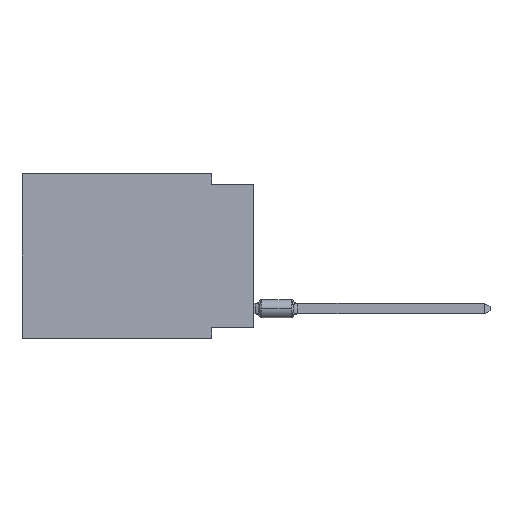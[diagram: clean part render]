
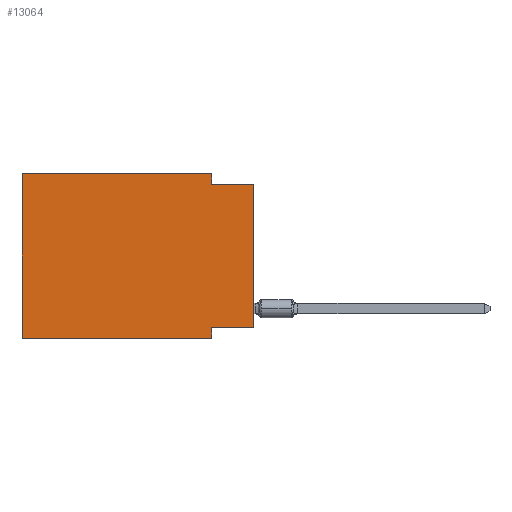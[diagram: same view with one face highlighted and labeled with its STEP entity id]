
A CAD part, left-side view. The second image highlights one B-rep face of the part: STEP entity #13064.
In plain terms, the highlighted planar face has unit normal (-1, 0, 0).
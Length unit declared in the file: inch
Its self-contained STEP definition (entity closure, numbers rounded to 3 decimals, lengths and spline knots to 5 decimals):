
#58 = VECTOR ( 'NONE', #435, 39.37008 ) ;
#290 = VECTOR ( 'NONE', #15337, 39.37008 ) ;
#435 = DIRECTION ( 'NONE',  ( 0., 0., -1. ) ) ;
#760 = DIRECTION ( 'NONE',  ( 0., 1., 0. ) ) ;
#1007 = DIRECTION ( 'NONE',  ( 0., -1., 0. ) ) ;
#1245 = ORIENTED_EDGE ( 'NONE', *, *, #11495, .T. ) ;
#1756 = ORIENTED_EDGE ( 'NONE', *, *, #4462, .F. ) ;
#1839 = DIRECTION ( 'NONE',  ( 0., 0., 1. ) ) ;
#2349 = LINE ( 'NONE', #4537, #13344 ) ;
#2824 = VECTOR ( 'NONE', #760, 39.37008 ) ;
#3099 = AXIS2_PLACEMENT_3D ( 'NONE', #5139, #9951, #13557 ) ;
#3325 = DIRECTION ( 'NONE',  ( 0., -1., 0. ) ) ;
#3511 = CARTESIAN_POINT ( 'NONE',  ( 0., 0.55, 0. ) ) ;
#4141 = ORIENTED_EDGE ( 'NONE', *, *, #4559, .F. ) ;
#4283 = CARTESIAN_POINT ( 'NONE',  ( 0., 0., -0.365 ) ) ;
#4462 = EDGE_CURVE ( 'NONE', #7658, #9899, #7679, .T. ) ;
#4537 = CARTESIAN_POINT ( 'NONE',  ( 0., 0.55, -0.39 ) ) ;
#4559 = EDGE_CURVE ( 'NONE', #5043, #13030, #5385, .T. ) ;
#4664 = ORIENTED_EDGE ( 'NONE', *, *, #12522, .F. ) ;
#5043 = VERTEX_POINT ( 'NONE', #10552 ) ;
#5113 = CARTESIAN_POINT ( 'NONE',  ( 0., 0., -0.025 ) ) ;
#5139 = CARTESIAN_POINT ( 'NONE',  ( 0., 0.55, 0. ) ) ;
#5385 = LINE ( 'NONE', #6409, #58 ) ;
#5472 = EDGE_LOOP ( 'NONE', ( #7021, #10696, #1756, #10956, #4664, #1245, #4141, #13862 ) ) ;
#5552 = VERTEX_POINT ( 'NONE', #8340 ) ;
#5589 = VECTOR ( 'NONE', #3325, 39.37008 ) ;
#6409 = CARTESIAN_POINT ( 'NONE',  ( 0., 0.1, -0.39 ) ) ;
#6539 = LINE ( 'NONE', #10310, #8101 ) ;
#6555 = CARTESIAN_POINT ( 'NONE',  ( 0., 0.55, 0. ) ) ;
#6660 = EDGE_CURVE ( 'NONE', #5552, #8252, #12189, .T. ) ;
#6736 = CARTESIAN_POINT ( 'NONE',  ( 0., 0.55, -0.39 ) ) ;
#7006 = VECTOR ( 'NONE', #14533, 39.37008 ) ;
#7021 = ORIENTED_EDGE ( 'NONE', *, *, #6660, .T. ) ;
#7084 = LINE ( 'NONE', #12830, #290 ) ;
#7658 = VERTEX_POINT ( 'NONE', #14203 ) ;
#7679 = LINE ( 'NONE', #7983, #14106 ) ;
#7983 = CARTESIAN_POINT ( 'NONE',  ( 0., 0.1, 0. ) ) ;
#8101 = VECTOR ( 'NONE', #1839, 39.37008 ) ;
#8252 = VERTEX_POINT ( 'NONE', #5113 ) ;
#8340 = CARTESIAN_POINT ( 'NONE',  ( 0., 0., -0.365 ) ) ;
#8657 = CARTESIAN_POINT ( 'NONE',  ( 0., 0., 0. ) ) ;
#9017 = DIRECTION ( 'NONE',  ( 0., 0., -1. ) ) ;
#9029 = LINE ( 'NONE', #4283, #2824 ) ;
#9684 = EDGE_CURVE ( 'NONE', #9899, #8252, #7084, .T. ) ;
#9899 = VERTEX_POINT ( 'NONE', #13448 ) ;
#9951 = DIRECTION ( 'NONE',  ( 1., 0., 0. ) ) ;
#10310 = CARTESIAN_POINT ( 'NONE',  ( 0., 0.55, 0. ) ) ;
#10552 = CARTESIAN_POINT ( 'NONE',  ( 0., 0.1, -0.365 ) ) ;
#10696 = ORIENTED_EDGE ( 'NONE', *, *, #9684, .F. ) ;
#10956 = ORIENTED_EDGE ( 'NONE', *, *, #15529, .F. ) ;
#11208 = PLANE ( 'NONE',  #3099 ) ;
#11486 = VERTEX_POINT ( 'NONE', #3511 ) ;
#11495 = EDGE_CURVE ( 'NONE', #11755, #13030, #2349, .T. ) ;
#11755 = VERTEX_POINT ( 'NONE', #6736 ) ;
#11780 = EDGE_CURVE ( 'NONE', #5552, #5043, #9029, .T. ) ;
#11933 = CARTESIAN_POINT ( 'NONE',  ( 0., 0.1, -0.39 ) ) ;
#12189 = LINE ( 'NONE', #8657, #7006 ) ;
#12522 = EDGE_CURVE ( 'NONE', #11755, #11486, #6539, .T. ) ;
#12830 = CARTESIAN_POINT ( 'NONE',  ( 0., 0., -0.025 ) ) ;
#13030 = VERTEX_POINT ( 'NONE', #11933 ) ;
#13064 = ADVANCED_FACE ( 'NONE', ( #14581 ), #11208, .F. ) ;
#13344 = VECTOR ( 'NONE', #1007, 39.37008 ) ;
#13448 = CARTESIAN_POINT ( 'NONE',  ( 0., 0.1, -0.025 ) ) ;
#13557 = DIRECTION ( 'NONE',  ( 0., 0., -1. ) ) ;
#13862 = ORIENTED_EDGE ( 'NONE', *, *, #11780, .F. ) ;
#14103 = LINE ( 'NONE', #6555, #5589 ) ;
#14106 = VECTOR ( 'NONE', #9017, 39.37008 ) ;
#14203 = CARTESIAN_POINT ( 'NONE',  ( 0., 0.1, 0. ) ) ;
#14533 = DIRECTION ( 'NONE',  ( 0., 0., 1. ) ) ;
#14581 = FACE_OUTER_BOUND ( 'NONE', #5472, .T. ) ;
#15337 = DIRECTION ( 'NONE',  ( 0., -1., 0. ) ) ;
#15529 = EDGE_CURVE ( 'NONE', #11486, #7658, #14103, .T. ) ;
